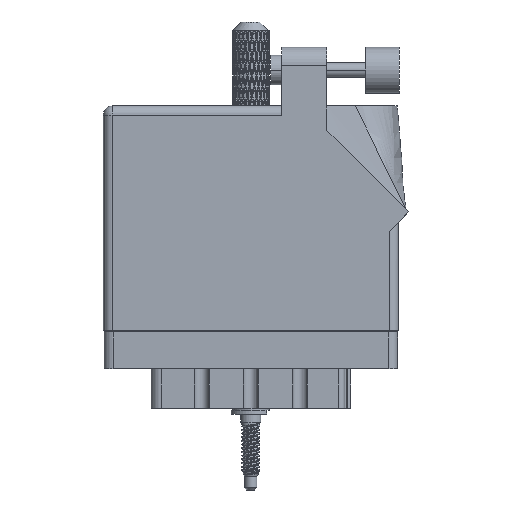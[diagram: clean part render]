
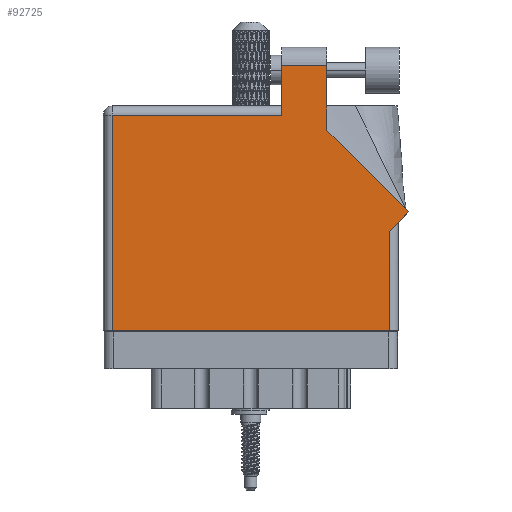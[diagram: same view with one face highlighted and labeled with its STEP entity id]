
A CAD part, front view. The second image highlights one B-rep face of the part: STEP entity #92725.
In plain terms, the highlighted face is planar.
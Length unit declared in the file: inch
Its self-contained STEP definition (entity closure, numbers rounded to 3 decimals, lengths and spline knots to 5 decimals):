
#494 = VECTOR ( 'NONE', #21723, 39.37008 ) ;
#5004 = ORIENTED_EDGE ( 'NONE', *, *, #32419, .T. ) ;
#6724 = ORIENTED_EDGE ( 'NONE', *, *, #33973, .T. ) ;
#7949 = VECTOR ( 'NONE', #99071, 39.37008 ) ;
#8326 = VECTOR ( 'NONE', #77594, 39.37008 ) ;
#9058 = ORIENTED_EDGE ( 'NONE', *, *, #96271, .T. ) ;
#9223 = ORIENTED_EDGE ( 'NONE', *, *, #40385, .T. ) ;
#10013 = DIRECTION ( 'NONE',  ( 0., 1., 0. ) ) ;
#10155 = CARTESIAN_POINT ( 'NONE',  ( 0., 1.468, 0. ) ) ;
#10949 = LINE ( 'NONE', #10155, #96177 ) ;
#12063 = VECTOR ( 'NONE', #82892, 39.37008 ) ;
#14499 = VERTEX_POINT ( 'NONE', #86750 ) ;
#16989 = CARTESIAN_POINT ( 'NONE',  ( 2.08071, 0.80771, 0. ) ) ;
#17112 = FACE_OUTER_BOUND ( 'NONE', #76908, .T. ) ;
#17137 = LINE ( 'NONE', #77966, #8326 ) ;
#19781 = VERTEX_POINT ( 'NONE', #16989 ) ;
#20960 = CARTESIAN_POINT ( 'NONE',  ( 1.948, 0.675, 0. ) ) ;
#21723 = DIRECTION ( 'NONE',  ( 1., 0., 0. ) ) ;
#22484 = LINE ( 'NONE', #87752, #494 ) ;
#23327 = DIRECTION ( 'NONE',  ( 0., -1., 0. ) ) ;
#24523 = VECTOR ( 'NONE', #43762, 39.37008 ) ;
#25152 = CARTESIAN_POINT ( 'NONE',  ( 1.948, 0.737, 0. ) ) ;
#27962 = EDGE_CURVE ( 'NONE', #19781, #89905, #17137, .T. ) ;
#29078 = EDGE_CURVE ( 'NONE', #60014, #75200, #84356, .T. ) ;
#32419 = EDGE_CURVE ( 'NONE', #89905, #60014, #82738, .T. ) ;
#33560 = CARTESIAN_POINT ( 'NONE',  ( 1.524, 1.805, 0. ) ) ;
#33973 = EDGE_CURVE ( 'NONE', #75200, #72344, #74877, .T. ) ;
#36264 = CARTESIAN_POINT ( 'NONE',  ( 1.217, 1.805, 0. ) ) ;
#36502 = ORIENTED_EDGE ( 'NONE', *, *, #58341, .T. ) ;
#36625 = DIRECTION ( 'NONE',  ( -1., 0., 0. ) ) ;
#39417 = PLANE ( 'NONE',  #67590 ) ;
#40385 = EDGE_CURVE ( 'NONE', #14499, #46924, #67691, .T. ) ;
#40393 = ORIENTED_EDGE ( 'NONE', *, *, #77047, .T. ) ;
#43762 = DIRECTION ( 'NONE',  ( 0., -1., 0. ) ) ;
#44445 = ORIENTED_EDGE ( 'NONE', *, *, #27962, .T. ) ;
#45724 = VECTOR ( 'NONE', #36625, 39.37008 ) ;
#46924 = VERTEX_POINT ( 'NONE', #20960 ) ;
#49210 = EDGE_CURVE ( 'NONE', #72344, #93006, #10949, .T. ) ;
#49263 = CARTESIAN_POINT ( 'NONE',  ( 1.217, 1.53, 0. ) ) ;
#54511 = CARTESIAN_POINT ( 'NONE',  ( 0.062, 0., 0. ) ) ;
#54869 = CARTESIAN_POINT ( 'NONE',  ( 0.062, 1.468, 0. ) ) ;
#58341 = EDGE_CURVE ( 'NONE', #46924, #19781, #95733, .T. ) ;
#60014 = VERTEX_POINT ( 'NONE', #33560 ) ;
#67590 = AXIS2_PLACEMENT_3D ( 'NONE', #104666, #103951, #88794 ) ;
#67691 = LINE ( 'NONE', #25152, #12063 ) ;
#72344 = VERTEX_POINT ( 'NONE', #78501 ) ;
#73478 = CARTESIAN_POINT ( 'NONE',  ( 0.062, 0., 0. ) ) ;
#74877 = LINE ( 'NONE', #49263, #24523 ) ;
#75200 = VERTEX_POINT ( 'NONE', #95872 ) ;
#75504 = DIRECTION ( 'NONE',  ( -1., 0., 0. ) ) ;
#76908 = EDGE_LOOP ( 'NONE', ( #5004, #102071, #6724, #103996, #40393, #9058, #9223, #36502, #44445 ) ) ;
#77047 = EDGE_CURVE ( 'NONE', #93006, #98571, #103083, .T. ) ;
#77594 = DIRECTION ( 'NONE',  ( -0.707, 0.707, 0. ) ) ;
#77966 = CARTESIAN_POINT ( 'NONE',  ( 2.08071, 0.80771, 0. ) ) ;
#78501 = CARTESIAN_POINT ( 'NONE',  ( 1.217, 1.468, 0. ) ) ;
#80174 = VECTOR ( 'NONE', #10013, 39.37008 ) ;
#82738 = LINE ( 'NONE', #100573, #80174 ) ;
#82892 = DIRECTION ( 'NONE',  ( 0., 1., 0. ) ) ;
#84356 = LINE ( 'NONE', #36264, #45724 ) ;
#86750 = CARTESIAN_POINT ( 'NONE',  ( 1.948, 0., 0. ) ) ;
#87752 = CARTESIAN_POINT ( 'NONE',  ( 0., 0., 0. ) ) ;
#88794 = DIRECTION ( 'NONE',  ( -1., 0., 0. ) ) ;
#89905 = VERTEX_POINT ( 'NONE', #93274 ) ;
#92725 = ADVANCED_FACE ( 'NONE', ( #17112 ), #39417, .F. ) ;
#93006 = VERTEX_POINT ( 'NONE', #54869 ) ;
#93274 = CARTESIAN_POINT ( 'NONE',  ( 1.524, 1.36442, 0. ) ) ;
#95733 = LINE ( 'NONE', #106284, #7949 ) ;
#95872 = CARTESIAN_POINT ( 'NONE',  ( 1.217, 1.805, 0. ) ) ;
#96177 = VECTOR ( 'NONE', #75504, 39.37008 ) ;
#96271 = EDGE_CURVE ( 'NONE', #98571, #14499, #22484, .T. ) ;
#98571 = VERTEX_POINT ( 'NONE', #54511 ) ;
#99071 = DIRECTION ( 'NONE',  ( 0.707, 0.707, 0. ) ) ;
#99272 = VECTOR ( 'NONE', #23327, 39.37008 ) ;
#100573 = CARTESIAN_POINT ( 'NONE',  ( 1.524, 1.36442, 0. ) ) ;
#102071 = ORIENTED_EDGE ( 'NONE', *, *, #29078, .T. ) ;
#103083 = LINE ( 'NONE', #73478, #99272 ) ;
#103951 = DIRECTION ( 'NONE',  ( 0., 0., -1. ) ) ;
#103996 = ORIENTED_EDGE ( 'NONE', *, *, #49210, .T. ) ;
#104666 = CARTESIAN_POINT ( 'NONE',  ( 0., 1.53, 0. ) ) ;
#106284 = CARTESIAN_POINT ( 'NONE',  ( 2.01, 0.737, 0. ) ) ;
